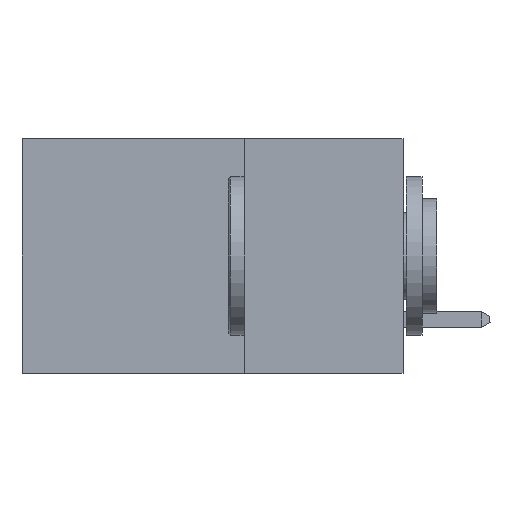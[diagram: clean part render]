
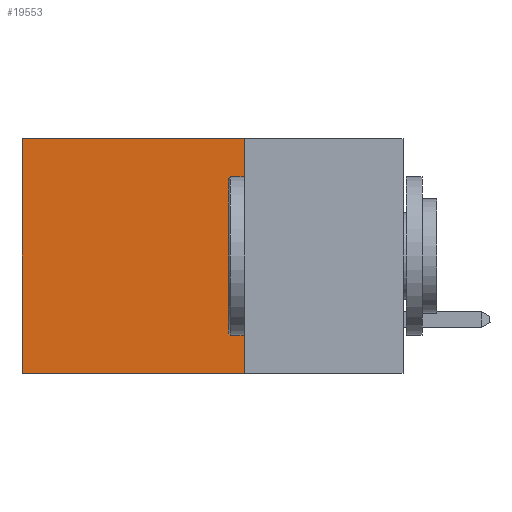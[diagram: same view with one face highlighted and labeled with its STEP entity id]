
A CAD part, left-side view. The second image highlights one B-rep face of the part: STEP entity #19553.
In plain terms, the highlighted planar face has unit normal (-1, 0, 0).
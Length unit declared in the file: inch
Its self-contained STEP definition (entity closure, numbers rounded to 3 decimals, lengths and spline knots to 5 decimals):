
#315 = DIRECTION ( 'NONE',  ( 1., 0., 0. ) ) ;
#431 = VERTEX_POINT ( 'NONE', #13469 ) ;
#2892 = VECTOR ( 'NONE', #28215, 39.37008 ) ;
#3773 = LINE ( 'NONE', #12771, #15406 ) ;
#4052 = CARTESIAN_POINT ( 'NONE',  ( 0.2875, 0.25, 0. ) ) ;
#4129 = LINE ( 'NONE', #4052, #8206 ) ;
#4152 = EDGE_CURVE ( 'NONE', #9739, #20815, #4129, .T. ) ;
#5685 = ORIENTED_EDGE ( 'NONE', *, *, #14224, .F. ) ;
#5914 = PLANE ( 'NONE',  #36323 ) ;
#6491 = CARTESIAN_POINT ( 'NONE',  ( 0.2875, 0.25, 0. ) ) ;
#8206 = VECTOR ( 'NONE', #24453, 39.37008 ) ;
#8262 = EDGE_CURVE ( 'NONE', #20815, #431, #3773, .T. ) ;
#8361 = CARTESIAN_POINT ( 'NONE',  ( 0.2875, 0.25, -0.37 ) ) ;
#9244 = EDGE_LOOP ( 'NONE', ( #16415, #5685, #27969, #26284 ) ) ;
#9394 = LINE ( 'NONE', #6491, #23328 ) ;
#9618 = DIRECTION ( 'NONE',  ( 0., 0., -1. ) ) ;
#9739 = VERTEX_POINT ( 'NONE', #27399 ) ;
#12083 = CARTESIAN_POINT ( 'NONE',  ( 0.2875, 0.6, 0. ) ) ;
#12654 = DIRECTION ( 'NONE',  ( 0., 0., -1. ) ) ;
#12771 = CARTESIAN_POINT ( 'NONE',  ( 0.2875, 0.6, 0. ) ) ;
#13469 = CARTESIAN_POINT ( 'NONE',  ( 0.2875, 0.6, -0.37 ) ) ;
#13532 = CARTESIAN_POINT ( 'NONE',  ( 0.2875, 0.25, -0.37 ) ) ;
#14224 = EDGE_CURVE ( 'NONE', #33166, #431, #19948, .T. ) ;
#15406 = VECTOR ( 'NONE', #12654, 39.37008 ) ;
#16415 = ORIENTED_EDGE ( 'NONE', *, *, #8262, .T. ) ;
#17541 = CARTESIAN_POINT ( 'NONE',  ( 0.2875, 0.25, 0. ) ) ;
#19553 = ADVANCED_FACE ( 'NONE', ( #21518 ), #5914, .F. ) ;
#19948 = LINE ( 'NONE', #8361, #2892 ) ;
#20430 = DIRECTION ( 'NONE',  ( 0., 0., -1. ) ) ;
#20815 = VERTEX_POINT ( 'NONE', #12083 ) ;
#21518 = FACE_OUTER_BOUND ( 'NONE', #9244, .T. ) ;
#23328 = VECTOR ( 'NONE', #9618, 39.37008 ) ;
#24453 = DIRECTION ( 'NONE',  ( 0., 1., 0. ) ) ;
#26284 = ORIENTED_EDGE ( 'NONE', *, *, #4152, .T. ) ;
#27399 = CARTESIAN_POINT ( 'NONE',  ( 0.2875, 0.25, 0. ) ) ;
#27969 = ORIENTED_EDGE ( 'NONE', *, *, #31746, .F. ) ;
#28215 = DIRECTION ( 'NONE',  ( 0., 1., 0. ) ) ;
#31746 = EDGE_CURVE ( 'NONE', #9739, #33166, #9394, .T. ) ;
#33166 = VERTEX_POINT ( 'NONE', #13532 ) ;
#36323 = AXIS2_PLACEMENT_3D ( 'NONE', #17541, #315, #20430 ) ;
